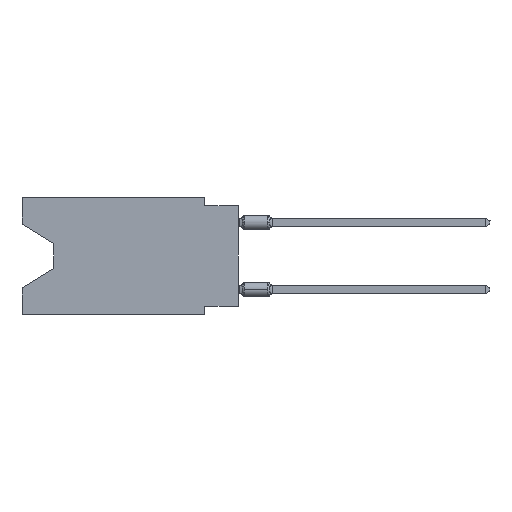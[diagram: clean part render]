
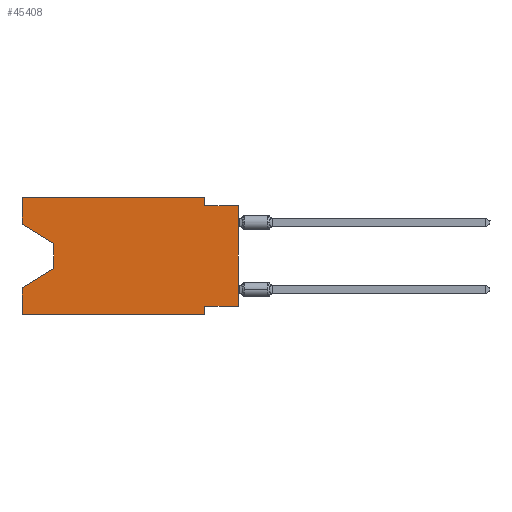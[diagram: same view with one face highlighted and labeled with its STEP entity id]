
A CAD part, left-side view. The second image highlights one B-rep face of the part: STEP entity #45408.
In plain terms, the highlighted planar face has unit normal (-1, 0, 0).
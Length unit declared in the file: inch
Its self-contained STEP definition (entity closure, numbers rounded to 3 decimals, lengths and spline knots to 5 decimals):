
#724 = EDGE_CURVE ( 'NONE', #60612, #65397, #38442, .T. ) ;
#2152 = ORIENTED_EDGE ( 'NONE', *, *, #43857, .F. ) ;
#2306 = LINE ( 'NONE', #35481, #43541 ) ;
#2554 = EDGE_CURVE ( 'NONE', #36740, #60998, #65938, .T. ) ;
#3291 = CARTESIAN_POINT ( 'NONE',  ( 0., 0., -0.025 ) ) ;
#4417 = EDGE_CURVE ( 'NONE', #26384, #14000, #57860, .T. ) ;
#4963 = LINE ( 'NONE', #16717, #61596 ) ;
#6032 = CARTESIAN_POINT ( 'NONE',  ( 0., 0.55, -0.212 ) ) ;
#6870 = CARTESIAN_POINT ( 'NONE',  ( 0., 0., 0. ) ) ;
#6918 = CARTESIAN_POINT ( 'NONE',  ( 0., 0., -0.325 ) ) ;
#7213 = DIRECTION ( 'NONE',  ( 0., 0., 1. ) ) ;
#9246 = CARTESIAN_POINT ( 'NONE',  ( 0., 0., -0.025 ) ) ;
#11709 = DIRECTION ( 'NONE',  ( 0., -0.855, -0.519 ) ) ;
#11931 = PLANE ( 'NONE',  #38065 ) ;
#14000 = VERTEX_POINT ( 'NONE', #9246 ) ;
#14122 = VECTOR ( 'NONE', #54839, 39.37008 ) ;
#14449 = VERTEX_POINT ( 'NONE', #45402 ) ;
#15010 = LINE ( 'NONE', #32148, #36813 ) ;
#16717 = CARTESIAN_POINT ( 'NONE',  ( 0., 0.645, -0.08025 ) ) ;
#17366 = CARTESIAN_POINT ( 'NONE',  ( 0., 0.645, -0.35 ) ) ;
#20076 = CARTESIAN_POINT ( 'NONE',  ( 0., 0., -0.325 ) ) ;
#20738 = VECTOR ( 'NONE', #43057, 39.37008 ) ;
#21643 = CARTESIAN_POINT ( 'NONE',  ( 0., 0.1, 0. ) ) ;
#22795 = VECTOR ( 'NONE', #25904, 39.37008 ) ;
#23084 = EDGE_CURVE ( 'NONE', #45231, #26384, #55155, .T. ) ;
#23456 = ORIENTED_EDGE ( 'NONE', *, *, #24024, .T. ) ;
#23945 = CARTESIAN_POINT ( 'NONE',  ( 0., 0.645, -0.35 ) ) ;
#24024 = EDGE_CURVE ( 'NONE', #44201, #14000, #24319, .T. ) ;
#24155 = VECTOR ( 'NONE', #33357, 39.37008 ) ;
#24252 = ORIENTED_EDGE ( 'NONE', *, *, #53124, .F. ) ;
#24319 = LINE ( 'NONE', #6870, #34536 ) ;
#24836 = DIRECTION ( 'NONE',  ( 0., 0., 1. ) ) ;
#25904 = DIRECTION ( 'NONE',  ( 0., 0., -1. ) ) ;
#26384 = VERTEX_POINT ( 'NONE', #33124 ) ;
#26730 = EDGE_CURVE ( 'NONE', #51145, #36740, #54796, .T. ) ;
#27324 = CARTESIAN_POINT ( 'NONE',  ( 0., 0.55, -0.138 ) ) ;
#27595 = EDGE_CURVE ( 'NONE', #36748, #51145, #4963, .T. ) ;
#27833 = ORIENTED_EDGE ( 'NONE', *, *, #27595, .T. ) ;
#30823 = DIRECTION ( 'NONE',  ( 0., 0., -1. ) ) ;
#31884 = VERTEX_POINT ( 'NONE', #39345 ) ;
#32148 = CARTESIAN_POINT ( 'NONE',  ( 0., 0.645, 0. ) ) ;
#33124 = CARTESIAN_POINT ( 'NONE',  ( 0., 0.1, -0.025 ) ) ;
#33357 = DIRECTION ( 'NONE',  ( 0., 1., 0. ) ) ;
#33700 = CARTESIAN_POINT ( 'NONE',  ( 0., 0.645, 0. ) ) ;
#34241 = CARTESIAN_POINT ( 'NONE',  ( 0., 0.55, -0.212 ) ) ;
#34536 = VECTOR ( 'NONE', #7213, 39.37008 ) ;
#35481 = CARTESIAN_POINT ( 'NONE',  ( 0., 0.1, -0.35 ) ) ;
#36740 = VERTEX_POINT ( 'NONE', #34241 ) ;
#36748 = VERTEX_POINT ( 'NONE', #62038 ) ;
#36813 = VECTOR ( 'NONE', #48526, 39.37008 ) ;
#37040 = CARTESIAN_POINT ( 'NONE',  ( 0., 0.1, 0. ) ) ;
#38065 = AXIS2_PLACEMENT_3D ( 'NONE', #33700, #62536, #67896 ) ;
#38442 = LINE ( 'NONE', #17366, #14122 ) ;
#39069 = FACE_OUTER_BOUND ( 'NONE', #58695, .T. ) ;
#39345 = CARTESIAN_POINT ( 'NONE',  ( 0., 0.645, 0. ) ) ;
#40655 = ORIENTED_EDGE ( 'NONE', *, *, #2554, .T. ) ;
#41572 = CARTESIAN_POINT ( 'NONE',  ( 0., 0.645, 0. ) ) ;
#41998 = VECTOR ( 'NONE', #56916, 39.37008 ) ;
#43057 = DIRECTION ( 'NONE',  ( 0., 0., -1. ) ) ;
#43541 = VECTOR ( 'NONE', #30823, 39.37008 ) ;
#43857 = EDGE_CURVE ( 'NONE', #31884, #45231, #67972, .T. ) ;
#44201 = VERTEX_POINT ( 'NONE', #20076 ) ;
#44961 = ORIENTED_EDGE ( 'NONE', *, *, #26730, .T. ) ;
#45231 = VERTEX_POINT ( 'NONE', #37040 ) ;
#45402 = CARTESIAN_POINT ( 'NONE',  ( 0., 0.1, -0.325 ) ) ;
#45408 = ADVANCED_FACE ( 'NONE', ( #39069 ), #11931, .F. ) ;
#46240 = ORIENTED_EDGE ( 'NONE', *, *, #4417, .F. ) ;
#48487 = DIRECTION ( 'NONE',  ( 0., 0.855, -0.519 ) ) ;
#48526 = DIRECTION ( 'NONE',  ( 0., 0., 1. ) ) ;
#51145 = VERTEX_POINT ( 'NONE', #67938 ) ;
#51325 = CARTESIAN_POINT ( 'NONE',  ( 0., 0.645, -0.26975 ) ) ;
#51443 = VECTOR ( 'NONE', #53231, 39.37008 ) ;
#53124 = EDGE_CURVE ( 'NONE', #36748, #31884, #56262, .T. ) ;
#53231 = DIRECTION ( 'NONE',  ( 0., -1., 0. ) ) ;
#53406 = ORIENTED_EDGE ( 'NONE', *, *, #59839, .F. ) ;
#54544 = VECTOR ( 'NONE', #24836, 39.37008 ) ;
#54796 = LINE ( 'NONE', #27324, #22795 ) ;
#54839 = DIRECTION ( 'NONE',  ( 0., -1., 0. ) ) ;
#55155 = LINE ( 'NONE', #21643, #20738 ) ;
#55840 = VECTOR ( 'NONE', #48487, 39.37008 ) ;
#56262 = LINE ( 'NONE', #62292, #54544 ) ;
#56916 = DIRECTION ( 'NONE',  ( 0., -1., 0. ) ) ;
#57860 = LINE ( 'NONE', #3291, #51443 ) ;
#58695 = EDGE_LOOP ( 'NONE', ( #27833, #44961, #40655, #69404, #61599, #53406, #69678, #23456, #46240, #68198, #2152, #24252 ) ) ;
#59839 = EDGE_CURVE ( 'NONE', #14449, #65397, #2306, .T. ) ;
#60021 = EDGE_CURVE ( 'NONE', #44201, #14449, #67190, .T. ) ;
#60612 = VERTEX_POINT ( 'NONE', #23945 ) ;
#60998 = VERTEX_POINT ( 'NONE', #51325 ) ;
#61596 = VECTOR ( 'NONE', #11709, 39.37008 ) ;
#61599 = ORIENTED_EDGE ( 'NONE', *, *, #724, .T. ) ;
#62038 = CARTESIAN_POINT ( 'NONE',  ( 0., 0.645, -0.08025 ) ) ;
#62292 = CARTESIAN_POINT ( 'NONE',  ( 0., 0.645, 0. ) ) ;
#62536 = DIRECTION ( 'NONE',  ( 1., 0., 0. ) ) ;
#65397 = VERTEX_POINT ( 'NONE', #70373 ) ;
#65938 = LINE ( 'NONE', #6032, #55840 ) ;
#67190 = LINE ( 'NONE', #6918, #24155 ) ;
#67726 = EDGE_CURVE ( 'NONE', #60612, #60998, #15010, .T. ) ;
#67896 = DIRECTION ( 'NONE',  ( 0., 0., -1. ) ) ;
#67938 = CARTESIAN_POINT ( 'NONE',  ( 0., 0.55, -0.138 ) ) ;
#67972 = LINE ( 'NONE', #41572, #41998 ) ;
#68198 = ORIENTED_EDGE ( 'NONE', *, *, #23084, .F. ) ;
#69404 = ORIENTED_EDGE ( 'NONE', *, *, #67726, .F. ) ;
#69678 = ORIENTED_EDGE ( 'NONE', *, *, #60021, .F. ) ;
#70373 = CARTESIAN_POINT ( 'NONE',  ( 0., 0.1, -0.35 ) ) ;
